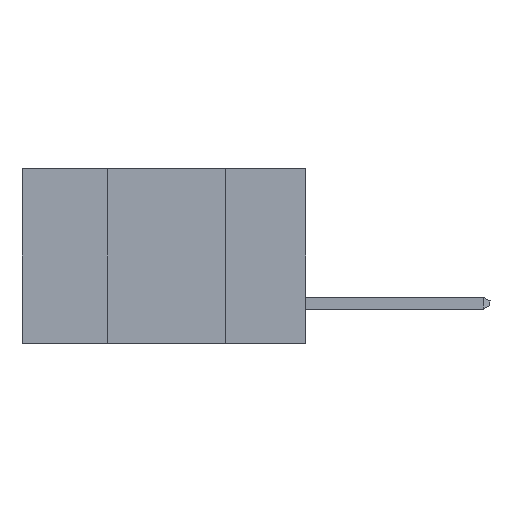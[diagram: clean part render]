
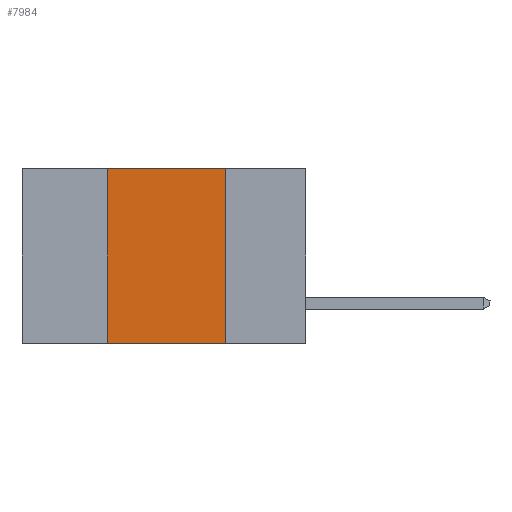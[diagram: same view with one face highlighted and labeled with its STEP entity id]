
A CAD part, left-side view. The second image highlights one B-rep face of the part: STEP entity #7984.
In plain terms, the highlighted planar face has unit normal (-1, 0, 0).
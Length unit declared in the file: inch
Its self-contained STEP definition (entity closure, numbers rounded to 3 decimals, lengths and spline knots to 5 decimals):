
#775 = VECTOR ( 'NONE', #20882, 39.37008 ) ;
#1284 = DIRECTION ( 'NONE',  ( 0., -1., 0. ) ) ;
#1518 = VERTEX_POINT ( 'NONE', #16060 ) ;
#1757 = VERTEX_POINT ( 'NONE', #13461 ) ;
#2013 = DIRECTION ( 'NONE',  ( 0., 0., -1. ) ) ;
#2033 = DIRECTION ( 'NONE',  ( 1., 0., 0. ) ) ;
#2056 = CARTESIAN_POINT ( 'NONE',  ( 0., 0.6, 0. ) ) ;
#2293 = PLANE ( 'NONE',  #6893 ) ;
#2707 = EDGE_CURVE ( 'NONE', #1757, #1518, #21228, .T. ) ;
#3216 = ORIENTED_EDGE ( 'NONE', *, *, #6311, .T. ) ;
#3381 = LINE ( 'NONE', #22754, #21969 ) ;
#4626 = EDGE_CURVE ( 'NONE', #1518, #22014, #3381, .T. ) ;
#4812 = FACE_OUTER_BOUND ( 'NONE', #14001, .T. ) ;
#6311 = EDGE_CURVE ( 'NONE', #1757, #16606, #13003, .T. ) ;
#6893 = AXIS2_PLACEMENT_3D ( 'NONE', #2056, #2033, #2013 ) ;
#7984 = ADVANCED_FACE ( 'NONE', ( #4812 ), #2293, .F. ) ;
#9840 = CARTESIAN_POINT ( 'NONE',  ( 0., 0.17, 0. ) ) ;
#10724 = DIRECTION ( 'NONE',  ( 0., 0., -1. ) ) ;
#10935 = VECTOR ( 'NONE', #10724, 39.37008 ) ;
#11523 = LINE ( 'NONE', #17850, #10935 ) ;
#13003 = LINE ( 'NONE', #19502, #17137 ) ;
#13128 = ORIENTED_EDGE ( 'NONE', *, *, #4626, .F. ) ;
#13461 = CARTESIAN_POINT ( 'NONE',  ( 0., 0.42, -0.37 ) ) ;
#14001 = EDGE_LOOP ( 'NONE', ( #18721, #13128, #16222, #3216 ) ) ;
#16060 = CARTESIAN_POINT ( 'NONE',  ( 0., 0.42, 0. ) ) ;
#16222 = ORIENTED_EDGE ( 'NONE', *, *, #2707, .F. ) ;
#16606 = VERTEX_POINT ( 'NONE', #22972 ) ;
#17137 = VECTOR ( 'NONE', #19532, 39.37008 ) ;
#17850 = CARTESIAN_POINT ( 'NONE',  ( 0., 0.17, -0.37 ) ) ;
#18721 = ORIENTED_EDGE ( 'NONE', *, *, #21683, .F. ) ;
#19502 = CARTESIAN_POINT ( 'NONE',  ( 0., 0.6, -0.37 ) ) ;
#19532 = DIRECTION ( 'NONE',  ( 0., -1., 0. ) ) ;
#20360 = CARTESIAN_POINT ( 'NONE',  ( 0., 0.42, -0.37 ) ) ;
#20882 = DIRECTION ( 'NONE',  ( 0., 0., 1. ) ) ;
#21228 = LINE ( 'NONE', #20360, #775 ) ;
#21683 = EDGE_CURVE ( 'NONE', #22014, #16606, #11523, .T. ) ;
#21969 = VECTOR ( 'NONE', #1284, 39.37008 ) ;
#22014 = VERTEX_POINT ( 'NONE', #9840 ) ;
#22754 = CARTESIAN_POINT ( 'NONE',  ( 0., 0.6, 0. ) ) ;
#22972 = CARTESIAN_POINT ( 'NONE',  ( 0., 0.17, -0.37 ) ) ;
